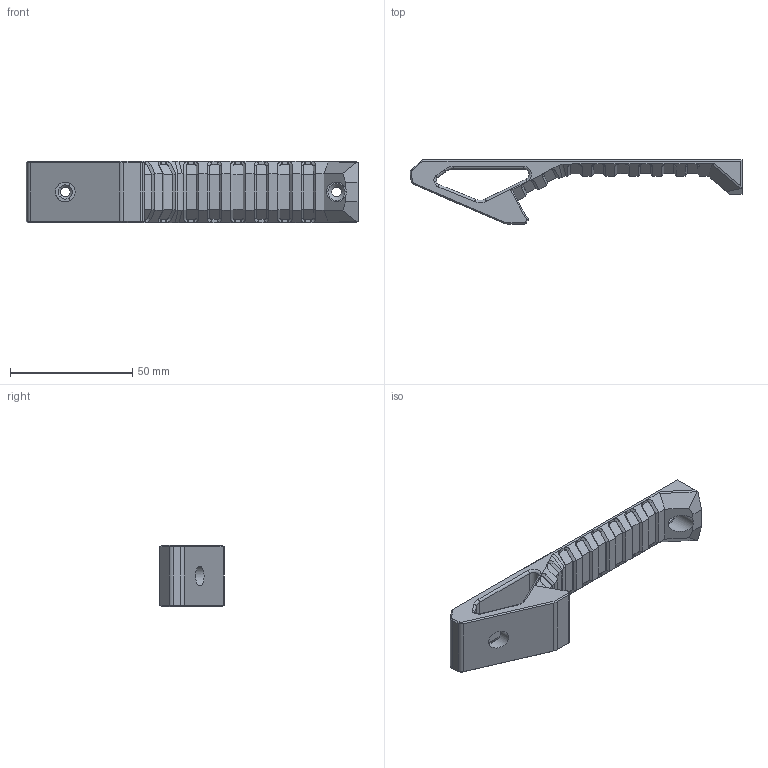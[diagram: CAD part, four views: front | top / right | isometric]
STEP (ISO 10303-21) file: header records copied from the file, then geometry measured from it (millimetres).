
FILE_DESCRIPTION(/* description */ (''),/* implementation_level */ '2;1');
FILE_NAME(/* name */ 'Large Hand Stop.step',/* time_stamp */ '2022-05-12T11:07:55-06:00',/* author */ (''),/* organization */ (''),/* preprocessor_version */ 'ST-DEVELOPER v18.1',/* originating_system */ 'Autodesk Translation Framework v10.10.0.1391',/* authorisation */ '');
FILE_SCHEMA (('AUTOMOTIVE_DESIGN { 1 0 10303 214 3 1 1 }'));
Length unit declared in the file: millimetre
Products named in the file (1): Hand stop 2
Bounding box: 135.82 x 26.2 x 25 mm (x, y, z)
Volume: 27624.2 mm3; surface area: 12153.1 mm2
Topology: 1 solids, 1 shells, 349 faces, 860 edges, 512 vertices
Faces by surface type: plane 194, cylinder 62, cone 47, bspline 36, torus 10
Full cylindrical faces by diameter (mm): 4 x2, 8.15 x2
Entity records: 10764 total; most frequent: CARTESIAN_POINT 2661, ORIENTED_EDGE 1720, DIRECTION 1598, EDGE_CURVE 860, LINE 600, VECTOR 600, VERTEX_POINT 512, AXIS2_PLACEMENT_3D 499
